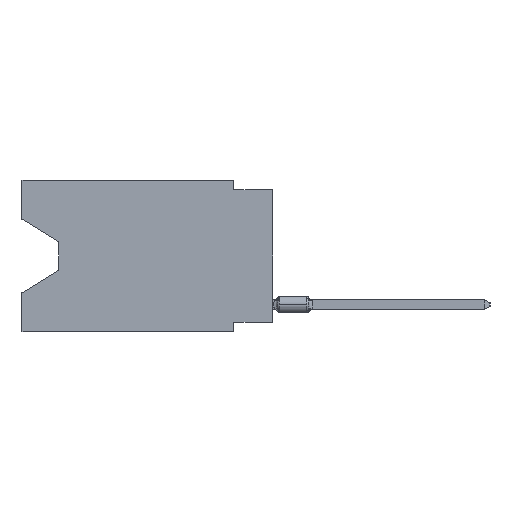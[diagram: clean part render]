
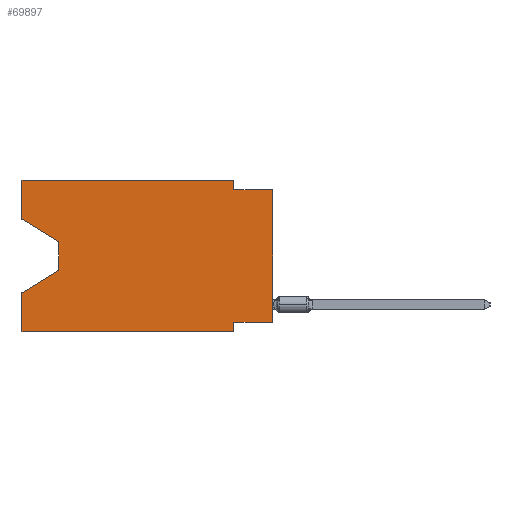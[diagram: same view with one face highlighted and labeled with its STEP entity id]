
A CAD part, left-side view. The second image highlights one B-rep face of the part: STEP entity #69897.
In plain terms, the highlighted planar face has unit normal (-1, 0, 0).
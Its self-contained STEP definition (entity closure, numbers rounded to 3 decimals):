
#1281 = LINE ( 'NONE', #25505, #37160 ) ;
#1544 = CARTESIAN_POINT ( 'NONE',  ( 0., 0., -0.635 ) ) ;
#3812 = VECTOR ( 'NONE', #17336, 1000. ) ;
#4038 = EDGE_CURVE ( 'NONE', #43192, #12114, #56339, .T. ) ;
#5759 = CARTESIAN_POINT ( 'NONE',  ( 0., 13.97, -5.893 ) ) ;
#5903 = EDGE_CURVE ( 'NONE', #10973, #34080, #47494, .T. ) ;
#6049 = ORIENTED_EDGE ( 'NONE', *, *, #32403, .T. ) ;
#8541 = DIRECTION ( 'NONE',  ( 0., 1., 0. ) ) ;
#8579 = CARTESIAN_POINT ( 'NONE',  ( 0., 16.383, 0. ) ) ;
#8900 = ORIENTED_EDGE ( 'NONE', *, *, #16013, .F. ) ;
#8932 = DIRECTION ( 'NONE',  ( 0., -1., 0. ) ) ;
#9000 = ORIENTED_EDGE ( 'NONE', *, *, #18355, .F. ) ;
#10810 = DIRECTION ( 'NONE',  ( 0., 0., 1. ) ) ;
#10973 = VERTEX_POINT ( 'NONE', #62681 ) ;
#11771 = VECTOR ( 'NONE', #39297, 1000. ) ;
#12114 = VERTEX_POINT ( 'NONE', #1544 ) ;
#12649 = VERTEX_POINT ( 'NONE', #40726 ) ;
#13483 = ORIENTED_EDGE ( 'NONE', *, *, #4038, .T. ) ;
#14125 = CARTESIAN_POINT ( 'NONE',  ( 0., 0., -9.271 ) ) ;
#15436 = CARTESIAN_POINT ( 'NONE',  ( 0., 0., 0. ) ) ;
#16013 = EDGE_CURVE ( 'NONE', #52851, #61714, #17867, .T. ) ;
#17336 = DIRECTION ( 'NONE',  ( 0., 0., 1. ) ) ;
#17867 = LINE ( 'NONE', #60564, #51541 ) ;
#18343 = CARTESIAN_POINT ( 'NONE',  ( 0., 16.383, -9.906 ) ) ;
#18355 = EDGE_CURVE ( 'NONE', #43192, #29994, #51436, .T. ) ;
#18772 = PLANE ( 'NONE',  #44065 ) ;
#19527 = CARTESIAN_POINT ( 'NONE',  ( 0., 16.383, -7.36 ) ) ;
#20635 = DIRECTION ( 'NONE',  ( 0., -0.855, -0.519 ) ) ;
#21258 = CARTESIAN_POINT ( 'NONE',  ( 0., 16.383, -9.906 ) ) ;
#22251 = ORIENTED_EDGE ( 'NONE', *, *, #72560, .F. ) ;
#23550 = FACE_OUTER_BOUND ( 'NONE', #76599, .T. ) ;
#24107 = EDGE_CURVE ( 'NONE', #61714, #12114, #48318, .T. ) ;
#25505 = CARTESIAN_POINT ( 'NONE',  ( 0., 13.97, -5.893 ) ) ;
#28673 = CARTESIAN_POINT ( 'NONE',  ( 0., 2.54, -0.635 ) ) ;
#29127 = VERTEX_POINT ( 'NONE', #5759 ) ;
#29994 = VERTEX_POINT ( 'NONE', #65365 ) ;
#30661 = CARTESIAN_POINT ( 'NONE',  ( 0., 16.383, 0. ) ) ;
#30780 = VERTEX_POINT ( 'NONE', #58025 ) ;
#32403 = EDGE_CURVE ( 'NONE', #12649, #29127, #33727, .T. ) ;
#32545 = LINE ( 'NONE', #75057, #53142 ) ;
#32845 = VECTOR ( 'NONE', #64636, 1000. ) ;
#33049 = VECTOR ( 'NONE', #8932, 1000. ) ;
#33557 = DIRECTION ( 'NONE',  ( 0., -1., 0. ) ) ;
#33727 = LINE ( 'NONE', #70278, #11771 ) ;
#34080 = VERTEX_POINT ( 'NONE', #8579 ) ;
#37160 = VECTOR ( 'NONE', #73967, 1000. ) ;
#38129 = EDGE_CURVE ( 'NONE', #10973, #12649, #32545, .T. ) ;
#39150 = VERTEX_POINT ( 'NONE', #18343 ) ;
#39198 = VECTOR ( 'NONE', #69841, 1000. ) ;
#39297 = DIRECTION ( 'NONE',  ( 0., 0., -1. ) ) ;
#39478 = ORIENTED_EDGE ( 'NONE', *, *, #67770, .T. ) ;
#40197 = VECTOR ( 'NONE', #33557, 1000. ) ;
#40726 = CARTESIAN_POINT ( 'NONE',  ( 0., 13.97, -4.013 ) ) ;
#40938 = ORIENTED_EDGE ( 'NONE', *, *, #61776, .F. ) ;
#41316 = ORIENTED_EDGE ( 'NONE', *, *, #61188, .F. ) ;
#42607 = DIRECTION ( 'NONE',  ( 0., 0., -1. ) ) ;
#43192 = VERTEX_POINT ( 'NONE', #52893 ) ;
#44065 = AXIS2_PLACEMENT_3D ( 'NONE', #30661, #72781, #42607 ) ;
#45587 = VECTOR ( 'NONE', #62788, 1000. ) ;
#46616 = CARTESIAN_POINT ( 'NONE',  ( 0., 2.54, 0. ) ) ;
#47494 = LINE ( 'NONE', #71730, #3812 ) ;
#48318 = LINE ( 'NONE', #72552, #32845 ) ;
#48811 = DIRECTION ( 'NONE',  ( 0., 0., -1. ) ) ;
#51436 = LINE ( 'NONE', #14125, #67083 ) ;
#51541 = VECTOR ( 'NONE', #48811, 1000. ) ;
#52851 = VERTEX_POINT ( 'NONE', #46616 ) ;
#52893 = CARTESIAN_POINT ( 'NONE',  ( 0., 0., -9.271 ) ) ;
#53142 = VECTOR ( 'NONE', #20635, 1000. ) ;
#55200 = ORIENTED_EDGE ( 'NONE', *, *, #24107, .F. ) ;
#55460 = ORIENTED_EDGE ( 'NONE', *, *, #5903, .F. ) ;
#56339 = LINE ( 'NONE', #15436, #39198 ) ;
#56975 = CARTESIAN_POINT ( 'NONE',  ( 0., 16.383, 0. ) ) ;
#57933 = EDGE_CURVE ( 'NONE', #39150, #30780, #64540, .T. ) ;
#58025 = CARTESIAN_POINT ( 'NONE',  ( 0., 2.54, -9.906 ) ) ;
#59241 = LINE ( 'NONE', #65223, #76337 ) ;
#60564 = CARTESIAN_POINT ( 'NONE',  ( 0., 2.54, 0. ) ) ;
#61188 = EDGE_CURVE ( 'NONE', #34080, #52851, #68912, .T. ) ;
#61714 = VERTEX_POINT ( 'NONE', #28673 ) ;
#61776 = EDGE_CURVE ( 'NONE', #39150, #72568, #59241, .T. ) ;
#62681 = CARTESIAN_POINT ( 'NONE',  ( 0., 16.383, -2.546 ) ) ;
#62788 = DIRECTION ( 'NONE',  ( 0., 0., -1. ) ) ;
#64540 = LINE ( 'NONE', #21258, #40197 ) ;
#64636 = DIRECTION ( 'NONE',  ( 0., -1., 0. ) ) ;
#65223 = CARTESIAN_POINT ( 'NONE',  ( 0., 16.383, 0. ) ) ;
#65365 = CARTESIAN_POINT ( 'NONE',  ( 0., 2.54, -9.271 ) ) ;
#67083 = VECTOR ( 'NONE', #8541, 1000. ) ;
#67770 = EDGE_CURVE ( 'NONE', #29127, #72568, #1281, .T. ) ;
#68090 = ORIENTED_EDGE ( 'NONE', *, *, #57933, .T. ) ;
#68912 = LINE ( 'NONE', #56975, #33049 ) ;
#69137 = CARTESIAN_POINT ( 'NONE',  ( 0., 2.54, -9.906 ) ) ;
#69841 = DIRECTION ( 'NONE',  ( 0., 0., 1. ) ) ;
#69897 = ADVANCED_FACE ( 'NONE', ( #23550 ), #18772, .F. ) ;
#70278 = CARTESIAN_POINT ( 'NONE',  ( 0., 13.97, -4.013 ) ) ;
#70316 = ORIENTED_EDGE ( 'NONE', *, *, #38129, .T. ) ;
#71730 = CARTESIAN_POINT ( 'NONE',  ( 0., 16.383, 0. ) ) ;
#72552 = CARTESIAN_POINT ( 'NONE',  ( 0., 0., -0.635 ) ) ;
#72560 = EDGE_CURVE ( 'NONE', #29994, #30780, #74323, .T. ) ;
#72568 = VERTEX_POINT ( 'NONE', #19527 ) ;
#72781 = DIRECTION ( 'NONE',  ( 1., 0., 0. ) ) ;
#73967 = DIRECTION ( 'NONE',  ( 0., 0.855, -0.519 ) ) ;
#74323 = LINE ( 'NONE', #69137, #45587 ) ;
#75057 = CARTESIAN_POINT ( 'NONE',  ( 0., 16.383, -2.546 ) ) ;
#76337 = VECTOR ( 'NONE', #10810, 1000. ) ;
#76599 = EDGE_LOOP ( 'NONE', ( #70316, #6049, #39478, #40938, #68090, #22251, #9000, #13483, #55200, #8900, #41316, #55460 ) ) ;
